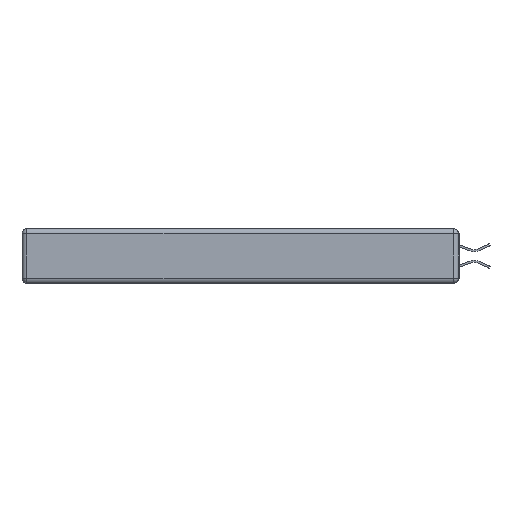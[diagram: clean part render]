
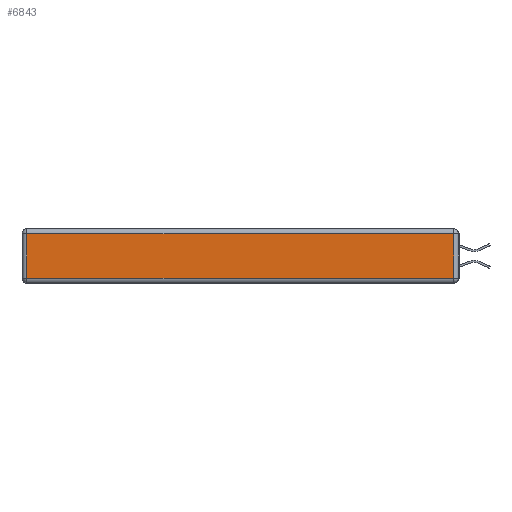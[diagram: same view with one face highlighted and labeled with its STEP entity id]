
A CAD part, left-side view. The second image highlights one B-rep face of the part: STEP entity #6843.
In plain terms, the highlighted planar face has unit normal (-1, 0, 0).
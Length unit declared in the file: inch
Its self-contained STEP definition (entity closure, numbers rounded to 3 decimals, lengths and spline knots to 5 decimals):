
#826 = CARTESIAN_POINT ( 'NONE',  ( 0., 2.72, -0.343 ) ) ;
#852 = ORIENTED_EDGE ( 'NONE', *, *, #13232, .T. ) ;
#1029 = EDGE_CURVE ( 'NONE', #10754, #11464, #15575, .T. ) ;
#1693 = CARTESIAN_POINT ( 'NONE',  ( 0., 0.03, -0.313 ) ) ;
#1941 = VERTEX_POINT ( 'NONE', #8296 ) ;
#2127 = ORIENTED_EDGE ( 'NONE', *, *, #1029, .T. ) ;
#2152 = AXIS2_PLACEMENT_3D ( 'NONE', #16285, #13714, #5960 ) ;
#2681 = CARTESIAN_POINT ( 'NONE',  ( 0., 0.03, -0.343 ) ) ;
#3676 = FACE_OUTER_BOUND ( 'NONE', #7673, .T. ) ;
#3865 = VECTOR ( 'NONE', #5722, 39.37008 ) ;
#4937 = CARTESIAN_POINT ( 'NONE',  ( 0., 2.72, -0.03 ) ) ;
#5425 = VECTOR ( 'NONE', #16590, 39.37008 ) ;
#5567 = CARTESIAN_POINT ( 'NONE',  ( 0., 2.75, -0.03 ) ) ;
#5722 = DIRECTION ( 'NONE',  ( 0., 0., -1. ) ) ;
#5944 = LINE ( 'NONE', #5567, #7560 ) ;
#5960 = DIRECTION ( 'NONE',  ( 0., 0., 1. ) ) ;
#6620 = DIRECTION ( 'NONE',  ( 0., 0., 1. ) ) ;
#6843 = ADVANCED_FACE ( 'NONE', ( #3676 ), #13593, .T. ) ;
#7334 = EDGE_CURVE ( 'NONE', #13160, #10754, #9475, .T. ) ;
#7560 = VECTOR ( 'NONE', #9401, 39.37008 ) ;
#7673 = EDGE_LOOP ( 'NONE', ( #2127, #852, #10471, #12841 ) ) ;
#8296 = CARTESIAN_POINT ( 'NONE',  ( 0., 0.03, -0.03 ) ) ;
#8304 = VECTOR ( 'NONE', #6620, 39.37008 ) ;
#9401 = DIRECTION ( 'NONE',  ( 0., 1., 0. ) ) ;
#9475 = LINE ( 'NONE', #826, #3865 ) ;
#10380 = EDGE_CURVE ( 'NONE', #1941, #13160, #5944, .T. ) ;
#10471 = ORIENTED_EDGE ( 'NONE', *, *, #10380, .T. ) ;
#10754 = VERTEX_POINT ( 'NONE', #12836 ) ;
#11464 = VERTEX_POINT ( 'NONE', #1693 ) ;
#12836 = CARTESIAN_POINT ( 'NONE',  ( 0., 2.72, -0.313 ) ) ;
#12841 = ORIENTED_EDGE ( 'NONE', *, *, #7334, .T. ) ;
#13160 = VERTEX_POINT ( 'NONE', #4937 ) ;
#13232 = EDGE_CURVE ( 'NONE', #11464, #1941, #15430, .T. ) ;
#13593 = PLANE ( 'NONE',  #2152 ) ;
#13714 = DIRECTION ( 'NONE',  ( -1., 0., 0. ) ) ;
#15430 = LINE ( 'NONE', #2681, #8304 ) ;
#15575 = LINE ( 'NONE', #16297, #5425 ) ;
#16285 = CARTESIAN_POINT ( 'NONE',  ( 0., 0., -0.343 ) ) ;
#16297 = CARTESIAN_POINT ( 'NONE',  ( 0., 0., -0.313 ) ) ;
#16590 = DIRECTION ( 'NONE',  ( 0., -1., 0. ) ) ;
